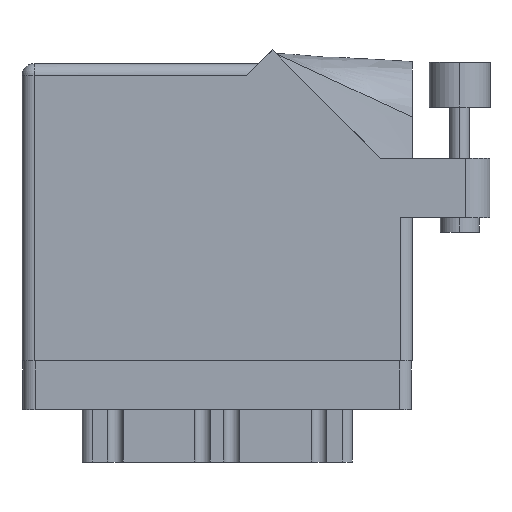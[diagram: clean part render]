
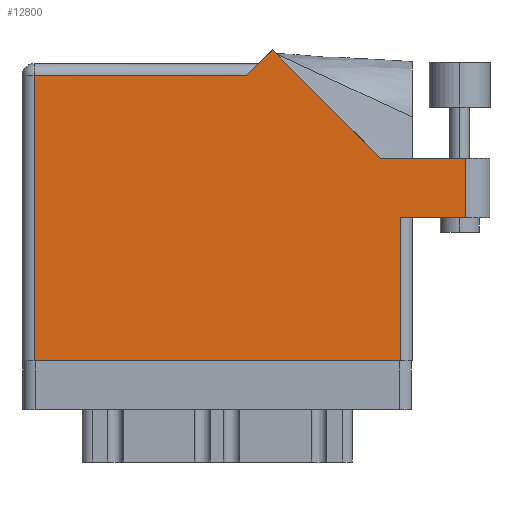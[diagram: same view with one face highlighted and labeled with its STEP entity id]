
A CAD part, front view. The second image highlights one B-rep face of the part: STEP entity #12800.
In plain terms, the highlighted face is planar.
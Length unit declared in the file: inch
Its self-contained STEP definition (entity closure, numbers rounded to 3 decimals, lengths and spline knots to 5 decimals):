
#567 = CARTESIAN_POINT ( 'NONE',  ( 0.062, 0., 0. ) ) ;
#896 = EDGE_CURVE ( 'NONE', #20814, #29735, #23564, .T. ) ;
#1419 = EDGE_CURVE ( 'NONE', #24873, #20814, #12377, .T. ) ;
#1500 = CARTESIAN_POINT ( 'NONE',  ( 1.28771, 1.60071, 0. ) ) ;
#1734 = ORIENTED_EDGE ( 'NONE', *, *, #8103, .T. ) ;
#2749 = VECTOR ( 'NONE', #9481, 39.37008 ) ;
#3317 = DIRECTION ( 'NONE',  ( 0., -1., 0. ) ) ;
#3785 = VERTEX_POINT ( 'NONE', #13692 ) ;
#5284 = LINE ( 'NONE', #27400, #27969 ) ;
#5362 = CARTESIAN_POINT ( 'NONE',  ( 0., 1.468, 0. ) ) ;
#5692 = VERTEX_POINT ( 'NONE', #7454 ) ;
#7141 = DIRECTION ( 'NONE',  ( -0.707, 0.707, 0. ) ) ;
#7454 = CARTESIAN_POINT ( 'NONE',  ( 1.84442, 1.044, 0. ) ) ;
#7781 = DIRECTION ( 'NONE',  ( -1., 0., 0. ) ) ;
#7840 = ORIENTED_EDGE ( 'NONE', *, *, #21686, .T. ) ;
#7858 = VERTEX_POINT ( 'NONE', #22146 ) ;
#7911 = LINE ( 'NONE', #5362, #8782 ) ;
#8103 = EDGE_CURVE ( 'NONE', #29735, #25205, #26262, .T. ) ;
#8782 = VECTOR ( 'NONE', #20264, 39.37008 ) ;
#9390 = LINE ( 'NONE', #567, #14427 ) ;
#9481 = DIRECTION ( 'NONE',  ( -0.707, -0.707, 0. ) ) ;
#11277 = AXIS2_PLACEMENT_3D ( 'NONE', #21895, #36973, #7781 ) ;
#11489 = ORIENTED_EDGE ( 'NONE', *, *, #19944, .T. ) ;
#12377 = LINE ( 'NONE', #36256, #32811 ) ;
#12800 = ADVANCED_FACE ( 'NONE', ( #22677 ), #34615, .F. ) ;
#12845 = ORIENTED_EDGE ( 'NONE', *, *, #28853, .T. ) ;
#13692 = CARTESIAN_POINT ( 'NONE',  ( 0.062, 0., 0. ) ) ;
#14427 = VECTOR ( 'NONE', #3317, 39.37008 ) ;
#15710 = CARTESIAN_POINT ( 'NONE',  ( 2.285, 1.044, 0. ) ) ;
#15786 = EDGE_LOOP ( 'NONE', ( #22447, #1734, #24003, #7840, #12845, #18398, #34604, #11489, #24274 ) ) ;
#17666 = CARTESIAN_POINT ( 'NONE',  ( 1.155, 1.468, 0. ) ) ;
#18398 = ORIENTED_EDGE ( 'NONE', *, *, #22123, .T. ) ;
#18750 = VECTOR ( 'NONE', #7141, 39.37008 ) ;
#19944 = EDGE_CURVE ( 'NONE', #3785, #24873, #5284, .T. ) ;
#20264 = DIRECTION ( 'NONE',  ( -1., 0., 0. ) ) ;
#20814 = VERTEX_POINT ( 'NONE', #33894 ) ;
#20820 = DIRECTION ( 'NONE',  ( 0., 1., 0. ) ) ;
#21686 = EDGE_CURVE ( 'NONE', #5692, #24851, #24398, .T. ) ;
#21694 = CARTESIAN_POINT ( 'NONE',  ( 1.948, 0., 0. ) ) ;
#21895 = CARTESIAN_POINT ( 'NONE',  ( 0., 1.53, 0. ) ) ;
#22123 = EDGE_CURVE ( 'NONE', #38160, #7858, #7911, .T. ) ;
#22146 = CARTESIAN_POINT ( 'NONE',  ( 0.062, 1.468, 0. ) ) ;
#22447 = ORIENTED_EDGE ( 'NONE', *, *, #896, .T. ) ;
#22677 = FACE_OUTER_BOUND ( 'NONE', #15786, .T. ) ;
#22787 = EDGE_CURVE ( 'NONE', #7858, #3785, #9390, .T. ) ;
#23564 = LINE ( 'NONE', #32563, #36791 ) ;
#24003 = ORIENTED_EDGE ( 'NONE', *, *, #31808, .T. ) ;
#24008 = LINE ( 'NONE', #35939, #2749 ) ;
#24217 = LINE ( 'NONE', #27152, #27984 ) ;
#24274 = ORIENTED_EDGE ( 'NONE', *, *, #1419, .T. ) ;
#24398 = LINE ( 'NONE', #28123, #18750 ) ;
#24851 = VERTEX_POINT ( 'NONE', #1500 ) ;
#24873 = VERTEX_POINT ( 'NONE', #21694 ) ;
#25205 = VERTEX_POINT ( 'NONE', #15710 ) ;
#25868 = VECTOR ( 'NONE', #26845, 39.37008 ) ;
#26262 = LINE ( 'NONE', #29767, #25868 ) ;
#26845 = DIRECTION ( 'NONE',  ( 0., 1., 0. ) ) ;
#27152 = CARTESIAN_POINT ( 'NONE',  ( 2.41, 1.044, 0. ) ) ;
#27400 = CARTESIAN_POINT ( 'NONE',  ( 0., 0., 0. ) ) ;
#27969 = VECTOR ( 'NONE', #33447, 39.37008 ) ;
#27984 = VECTOR ( 'NONE', #32827, 39.37008 ) ;
#28123 = CARTESIAN_POINT ( 'NONE',  ( 1.84442, 1.044, 0. ) ) ;
#28853 = EDGE_CURVE ( 'NONE', #24851, #38160, #24008, .T. ) ;
#29735 = VERTEX_POINT ( 'NONE', #32727 ) ;
#29767 = CARTESIAN_POINT ( 'NONE',  ( 2.285, 1.044, 0. ) ) ;
#31808 = EDGE_CURVE ( 'NONE', #25205, #5692, #24217, .T. ) ;
#32372 = DIRECTION ( 'NONE',  ( 1., 0., 0. ) ) ;
#32563 = CARTESIAN_POINT ( 'NONE',  ( 2.01, 0.737, 0. ) ) ;
#32727 = CARTESIAN_POINT ( 'NONE',  ( 2.285, 0.737, 0. ) ) ;
#32811 = VECTOR ( 'NONE', #20820, 39.37008 ) ;
#32827 = DIRECTION ( 'NONE',  ( -1., 0., 0. ) ) ;
#33447 = DIRECTION ( 'NONE',  ( 1., 0., 0. ) ) ;
#33894 = CARTESIAN_POINT ( 'NONE',  ( 1.948, 0.737, 0. ) ) ;
#34604 = ORIENTED_EDGE ( 'NONE', *, *, #22787, .T. ) ;
#34615 = PLANE ( 'NONE',  #11277 ) ;
#35939 = CARTESIAN_POINT ( 'NONE',  ( 1.217, 1.53, 0. ) ) ;
#36256 = CARTESIAN_POINT ( 'NONE',  ( 1.948, 0.737, 0. ) ) ;
#36791 = VECTOR ( 'NONE', #32372, 39.37008 ) ;
#36973 = DIRECTION ( 'NONE',  ( 0., 0., -1. ) ) ;
#38160 = VERTEX_POINT ( 'NONE', #17666 ) ;
